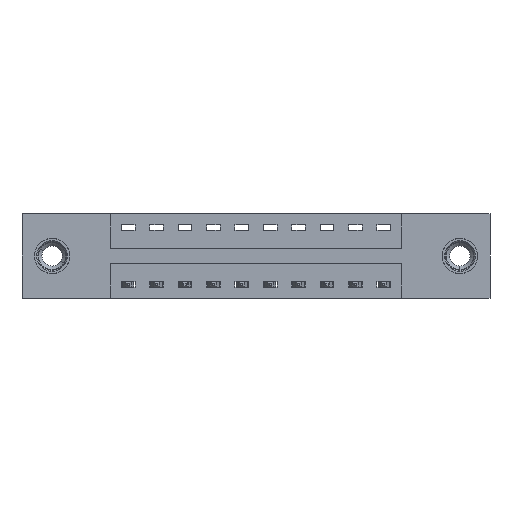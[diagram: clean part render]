
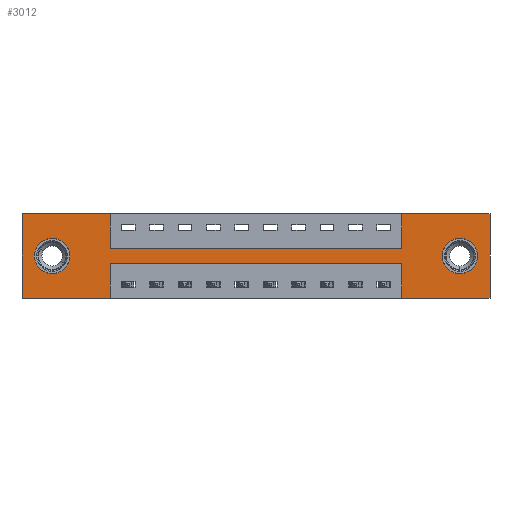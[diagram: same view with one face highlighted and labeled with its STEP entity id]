
A CAD part, front view. The second image highlights one B-rep face of the part: STEP entity #3012.
In plain terms, the highlighted planar face has unit normal (0, -1, 0).
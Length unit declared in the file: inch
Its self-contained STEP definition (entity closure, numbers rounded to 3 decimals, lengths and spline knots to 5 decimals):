
#24 = AXIS2_PLACEMENT_3D ( 'NONE', #5227, #719, #4244 ) ;
#29 = EDGE_CURVE ( 'NONE', #4252, #11254, #6775, .T. ) ;
#238 = DIRECTION ( 'NONE',  ( -1., 0., 0. ) ) ;
#280 = LINE ( 'NONE', #3903, #7705 ) ;
#417 = PLANE ( 'NONE',  #809 ) ;
#427 = CIRCLE ( 'NONE', #8547, 0.078 ) ;
#498 = ORIENTED_EDGE ( 'NONE', *, *, #8518, .F. ) ;
#598 = VERTEX_POINT ( 'NONE', #3381 ) ;
#630 = ORIENTED_EDGE ( 'NONE', *, *, #9134, .F. ) ;
#668 = ORIENTED_EDGE ( 'NONE', *, *, #5331, .F. ) ;
#719 = DIRECTION ( 'NONE',  ( 0., 1., 0. ) ) ;
#809 = AXIS2_PLACEMENT_3D ( 'NONE', #10273, #2288, #8407 ) ;
#833 = CARTESIAN_POINT ( 'NONE',  ( 0., 0., 0. ) ) ;
#884 = EDGE_CURVE ( 'NONE', #11254, #598, #10435, .T. ) ;
#982 = VECTOR ( 'NONE', #6312, 39.37008 ) ;
#1205 = VERTEX_POINT ( 'NONE', #4845 ) ;
#1347 = ORIENTED_EDGE ( 'NONE', *, *, #3026, .F. ) ;
#1539 = VECTOR ( 'NONE', #10418, 39.37008 ) ;
#1838 = DIRECTION ( 'NONE',  ( 0., 0., 1. ) ) ;
#1847 = CARTESIAN_POINT ( 'NONE',  ( 0.1325, 0., -0.185 ) ) ;
#2039 = CARTESIAN_POINT ( 'NONE',  ( 0., 0., -0.37 ) ) ;
#2107 = ORIENTED_EDGE ( 'NONE', *, *, #8622, .F. ) ;
#2112 = CARTESIAN_POINT ( 'NONE',  ( 0.1325, 0., -0.185 ) ) ;
#2117 = CIRCLE ( 'NONE', #24, 0.078 ) ;
#2187 = FACE_OUTER_BOUND ( 'NONE', #3423, .T. ) ;
#2237 = CARTESIAN_POINT ( 'NONE',  ( 0.3875, 0., -0.22 ) ) ;
#2288 = DIRECTION ( 'NONE',  ( 0., -1., 0. ) ) ;
#2315 = CARTESIAN_POINT ( 'NONE',  ( 1.6725, 0., 0. ) ) ;
#2398 = EDGE_CURVE ( 'NONE', #3535, #9873, #2815, .T. ) ;
#2424 = DIRECTION ( 'NONE',  ( 0., 0., 1. ) ) ;
#2540 = DIRECTION ( 'NONE',  ( 0., 0., 1. ) ) ;
#2605 = VECTOR ( 'NONE', #1838, 39.37008 ) ;
#2644 = VECTOR ( 'NONE', #4548, 39.37008 ) ;
#2684 = VERTEX_POINT ( 'NONE', #10349 ) ;
#2694 = VECTOR ( 'NONE', #6269, 39.37008 ) ;
#2815 = LINE ( 'NONE', #8881, #982 ) ;
#3012 = ADVANCED_FACE ( 'NONE', ( #6745, #9371, #2187 ), #417, .T. ) ;
#3026 = EDGE_CURVE ( 'NONE', #598, #10447, #10385, .T. ) ;
#3145 = DIRECTION ( 'NONE',  ( 1., 0., 0. ) ) ;
#3210 = LINE ( 'NONE', #11285, #8383 ) ;
#3381 = CARTESIAN_POINT ( 'NONE',  ( 1.6725, 0., -0.22 ) ) ;
#3423 = EDGE_LOOP ( 'NONE', ( #4298, #1347, #9368, #10553, #9467, #2107, #668, #630, #8442, #498, #6788, #3899 ) ) ;
#3458 = EDGE_CURVE ( 'NONE', #11589, #11433, #7246, .T. ) ;
#3506 = DIRECTION ( 'NONE',  ( 0., 1., 0. ) ) ;
#3535 = VERTEX_POINT ( 'NONE', #8324 ) ;
#3739 = AXIS2_PLACEMENT_3D ( 'NONE', #1847, #3506, #2540 ) ;
#3760 = CARTESIAN_POINT ( 'NONE',  ( 2.06, 0., 0. ) ) ;
#3899 = ORIENTED_EDGE ( 'NONE', *, *, #2398, .F. ) ;
#3903 = CARTESIAN_POINT ( 'NONE',  ( 0.3875, 0., -0.37 ) ) ;
#4148 = VECTOR ( 'NONE', #9823, 39.37008 ) ;
#4160 = CARTESIAN_POINT ( 'NONE',  ( 2.06, 0., -0.37 ) ) ;
#4244 = DIRECTION ( 'NONE',  ( 0., 0., -1. ) ) ;
#4252 = VERTEX_POINT ( 'NONE', #4160 ) ;
#4298 = ORIENTED_EDGE ( 'NONE', *, *, #8240, .F. ) ;
#4335 = VERTEX_POINT ( 'NONE', #5142 ) ;
#4546 = VECTOR ( 'NONE', #7603, 39.37008 ) ;
#4548 = DIRECTION ( 'NONE',  ( 0., 0., -1. ) ) ;
#4643 = CARTESIAN_POINT ( 'NONE',  ( 1.9275, 0., -0.263 ) ) ;
#4757 = VERTEX_POINT ( 'NONE', #4969 ) ;
#4845 = CARTESIAN_POINT ( 'NONE',  ( 2.06, 0., 0. ) ) ;
#4870 = VERTEX_POINT ( 'NONE', #9647 ) ;
#4906 = CARTESIAN_POINT ( 'NONE',  ( 0.1325, 0., -0.107 ) ) ;
#4969 = CARTESIAN_POINT ( 'NONE',  ( 0.3875, 0., -0.15 ) ) ;
#5005 = EDGE_CURVE ( 'NONE', #1205, #4252, #10942, .T. ) ;
#5110 = CARTESIAN_POINT ( 'NONE',  ( 0.3875, 0., -0.22 ) ) ;
#5142 = CARTESIAN_POINT ( 'NONE',  ( 1.9275, 0., -0.107 ) ) ;
#5227 = CARTESIAN_POINT ( 'NONE',  ( 1.9275, 0., -0.185 ) ) ;
#5301 = EDGE_CURVE ( 'NONE', #4335, #10791, #2117, .T. ) ;
#5331 = EDGE_CURVE ( 'NONE', #2684, #8878, #8664, .T. ) ;
#5590 = EDGE_CURVE ( 'NONE', #10791, #4335, #427, .T. ) ;
#5677 = VECTOR ( 'NONE', #5731, 39.37008 ) ;
#5731 = DIRECTION ( 'NONE',  ( 0., 0., 1. ) ) ;
#5785 = EDGE_LOOP ( 'NONE', ( #8494, #11073 ) ) ;
#6269 = DIRECTION ( 'NONE',  ( 0., 0., -1. ) ) ;
#6292 = CARTESIAN_POINT ( 'NONE',  ( 0.3875, 0., 0. ) ) ;
#6312 = DIRECTION ( 'NONE',  ( -1., 0., 0. ) ) ;
#6473 = CARTESIAN_POINT ( 'NONE',  ( 0., 0., 0. ) ) ;
#6580 = EDGE_CURVE ( 'NONE', #8516, #4757, #7464, .T. ) ;
#6709 = DIRECTION ( 'NONE',  ( 0., 0., -1. ) ) ;
#6725 = CARTESIAN_POINT ( 'NONE',  ( 0., 0., -0.37 ) ) ;
#6745 = FACE_BOUND ( 'NONE', #5785, .T. ) ;
#6775 = LINE ( 'NONE', #2039, #1539 ) ;
#6788 = ORIENTED_EDGE ( 'NONE', *, *, #11632, .F. ) ;
#7203 = VECTOR ( 'NONE', #2424, 39.37008 ) ;
#7229 = CARTESIAN_POINT ( 'NONE',  ( 1.6725, 0., 0. ) ) ;
#7246 = CIRCLE ( 'NONE', #11252, 0.078 ) ;
#7448 = ORIENTED_EDGE ( 'NONE', *, *, #10223, .T. ) ;
#7464 = LINE ( 'NONE', #11107, #2694 ) ;
#7492 = ORIENTED_EDGE ( 'NONE', *, *, #3458, .T. ) ;
#7500 = DIRECTION ( 'NONE',  ( 0., 0., -1. ) ) ;
#7603 = DIRECTION ( 'NONE',  ( 1., 0., 0. ) ) ;
#7705 = VECTOR ( 'NONE', #7500, 39.37008 ) ;
#8240 = EDGE_CURVE ( 'NONE', #10447, #3535, #280, .T. ) ;
#8266 = CIRCLE ( 'NONE', #3739, 0.078 ) ;
#8314 = EDGE_LOOP ( 'NONE', ( #7448, #7492 ) ) ;
#8324 = CARTESIAN_POINT ( 'NONE',  ( 0.3875, 0., -0.37 ) ) ;
#8383 = VECTOR ( 'NONE', #3145, 39.37008 ) ;
#8407 = DIRECTION ( 'NONE',  ( 0., 0., -1. ) ) ;
#8442 = ORIENTED_EDGE ( 'NONE', *, *, #6580, .F. ) ;
#8494 = ORIENTED_EDGE ( 'NONE', *, *, #5301, .T. ) ;
#8516 = VERTEX_POINT ( 'NONE', #6292 ) ;
#8518 = EDGE_CURVE ( 'NONE', #4870, #8516, #10703, .T. ) ;
#8547 = AXIS2_PLACEMENT_3D ( 'NONE', #11232, #9326, #6709 ) ;
#8622 = EDGE_CURVE ( 'NONE', #8878, #1205, #10127, .T. ) ;
#8664 = LINE ( 'NONE', #2315, #7203 ) ;
#8688 = CARTESIAN_POINT ( 'NONE',  ( 1.6725, 0., -0.37 ) ) ;
#8878 = VERTEX_POINT ( 'NONE', #7229 ) ;
#8881 = CARTESIAN_POINT ( 'NONE',  ( 0., 0., -0.37 ) ) ;
#8981 = CARTESIAN_POINT ( 'NONE',  ( 0., 0., 0. ) ) ;
#9134 = EDGE_CURVE ( 'NONE', #4757, #2684, #3210, .T. ) ;
#9326 = DIRECTION ( 'NONE',  ( 0., 1., 0. ) ) ;
#9368 = ORIENTED_EDGE ( 'NONE', *, *, #884, .F. ) ;
#9371 = FACE_BOUND ( 'NONE', #8314, .T. ) ;
#9467 = ORIENTED_EDGE ( 'NONE', *, *, #5005, .F. ) ;
#9485 = CARTESIAN_POINT ( 'NONE',  ( 1.6725, 0., -0.37 ) ) ;
#9647 = CARTESIAN_POINT ( 'NONE',  ( 0., 0., 0. ) ) ;
#9746 = CARTESIAN_POINT ( 'NONE',  ( 0.1325, 0., -0.263 ) ) ;
#9823 = DIRECTION ( 'NONE',  ( 1., 0., 0. ) ) ;
#9873 = VERTEX_POINT ( 'NONE', #6725 ) ;
#10127 = LINE ( 'NONE', #6473, #4546 ) ;
#10196 = DIRECTION ( 'NONE',  ( 0., 0., 1. ) ) ;
#10223 = EDGE_CURVE ( 'NONE', #11433, #11589, #8266, .T. ) ;
#10273 = CARTESIAN_POINT ( 'NONE',  ( 0., 0., -0.37 ) ) ;
#10349 = CARTESIAN_POINT ( 'NONE',  ( 1.6725, 0., -0.15 ) ) ;
#10385 = LINE ( 'NONE', #2237, #11611 ) ;
#10418 = DIRECTION ( 'NONE',  ( -1., 0., 0. ) ) ;
#10435 = LINE ( 'NONE', #9485, #5677 ) ;
#10447 = VERTEX_POINT ( 'NONE', #5110 ) ;
#10553 = ORIENTED_EDGE ( 'NONE', *, *, #29, .F. ) ;
#10703 = LINE ( 'NONE', #8981, #4148 ) ;
#10791 = VERTEX_POINT ( 'NONE', #4643 ) ;
#10942 = LINE ( 'NONE', #3760, #2644 ) ;
#11073 = ORIENTED_EDGE ( 'NONE', *, *, #5590, .T. ) ;
#11107 = CARTESIAN_POINT ( 'NONE',  ( 0.3875, 0., 0. ) ) ;
#11200 = DIRECTION ( 'NONE',  ( 0., 1., 0. ) ) ;
#11232 = CARTESIAN_POINT ( 'NONE',  ( 1.9275, 0., -0.185 ) ) ;
#11252 = AXIS2_PLACEMENT_3D ( 'NONE', #2112, #11200, #10196 ) ;
#11254 = VERTEX_POINT ( 'NONE', #8688 ) ;
#11285 = CARTESIAN_POINT ( 'NONE',  ( 0.3875, 0., -0.15 ) ) ;
#11433 = VERTEX_POINT ( 'NONE', #4906 ) ;
#11589 = VERTEX_POINT ( 'NONE', #9746 ) ;
#11611 = VECTOR ( 'NONE', #238, 39.37008 ) ;
#11632 = EDGE_CURVE ( 'NONE', #9873, #4870, #11633, .T. ) ;
#11633 = LINE ( 'NONE', #833, #2605 ) ;
